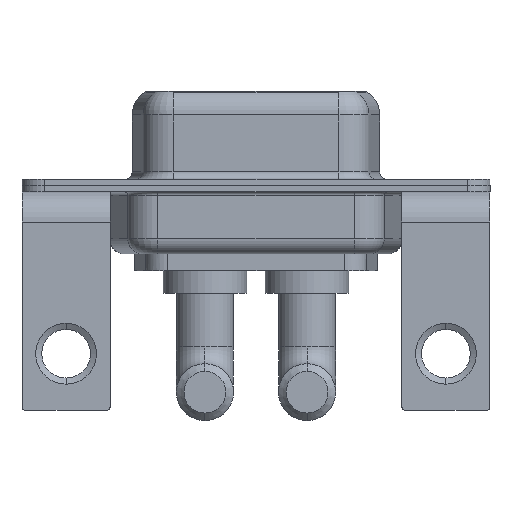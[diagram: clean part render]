
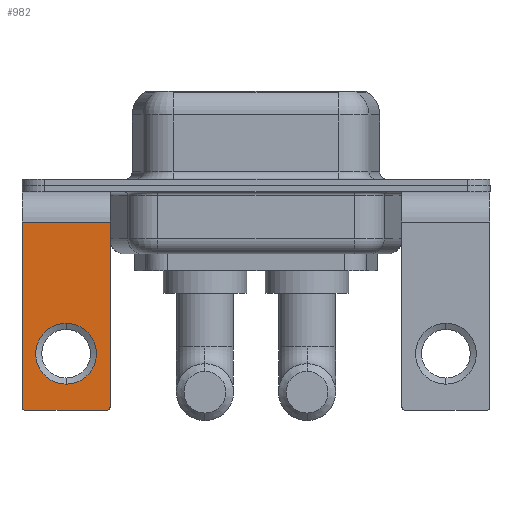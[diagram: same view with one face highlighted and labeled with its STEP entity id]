
A CAD part, front view. The second image highlights one B-rep face of the part: STEP entity #982.
In plain terms, the highlighted planar face has unit normal (0, -1, 0).
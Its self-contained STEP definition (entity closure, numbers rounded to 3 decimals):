
#19 = VERTEX_POINT ( 'NONE', #1839 ) ;
#509 = VECTOR ( 'NONE', #10848, 1000. ) ;
#629 = LINE ( 'NONE', #2600, #3010 ) ;
#982 = ADVANCED_FACE ( 'NONE', ( #2645, #2837 ), #10839, .F. ) ;
#1066 = ORIENTED_EDGE ( 'NONE', *, *, #7491, .F. ) ;
#1221 = ORIENTED_EDGE ( 'NONE', *, *, #5787, .T. ) ;
#1778 = EDGE_LOOP ( 'NONE', ( #9861, #5299, #6049, #1221, #1066, #8559 ) ) ;
#1783 = DIRECTION ( 'NONE',  ( 0., 1., 0. ) ) ;
#1839 = CARTESIAN_POINT ( 'NONE',  ( -2.9, -6.25, -2.4 ) ) ;
#1946 = CARTESIAN_POINT ( 'NONE',  ( 2.65, -6.25, -14.55 ) ) ;
#2063 = DIRECTION ( 'NONE',  ( 0., 0., 1. ) ) ;
#2127 = DIRECTION ( 'NONE',  ( -1., 0., 0. ) ) ;
#2351 = CARTESIAN_POINT ( 'NONE',  ( 0., -6.25, -11.07 ) ) ;
#2417 = CARTESIAN_POINT ( 'NONE',  ( -2.9, -6.25, -14.55 ) ) ;
#2541 = CARTESIAN_POINT ( 'NONE',  ( 2.9, -6.25, -14.55 ) ) ;
#2587 = EDGE_CURVE ( 'NONE', #19, #12319, #629, .T. ) ;
#2600 = CARTESIAN_POINT ( 'NONE',  ( -2.9, -6.25, -2.4 ) ) ;
#2645 = FACE_BOUND ( 'NONE', #3706, .T. ) ;
#2831 = CARTESIAN_POINT ( 'NONE',  ( 0., -6.25, -13.07 ) ) ;
#2837 = FACE_OUTER_BOUND ( 'NONE', #1778, .T. ) ;
#3010 = VECTOR ( 'NONE', #6517, 1000. ) ;
#3052 = DIRECTION ( 'NONE',  ( 0., -1., 0. ) ) ;
#3208 = CIRCLE ( 'NONE', #12373, 0.25 ) ;
#3221 = LINE ( 'NONE', #9207, #9696 ) ;
#3277 = AXIS2_PLACEMENT_3D ( 'NONE', #2351, #10372, #4375 ) ;
#3706 = EDGE_LOOP ( 'NONE', ( #7276, #4104 ) ) ;
#4031 = CARTESIAN_POINT ( 'NONE',  ( -2.65, -6.25, -14.55 ) ) ;
#4104 = ORIENTED_EDGE ( 'NONE', *, *, #11222, .T. ) ;
#4375 = DIRECTION ( 'NONE',  ( 0., 0., 1. ) ) ;
#5279 = CIRCLE ( 'NONE', #9665, 0.25 ) ;
#5299 = ORIENTED_EDGE ( 'NONE', *, *, #6335, .T. ) ;
#5304 = DIRECTION ( 'NONE',  ( 0., 0., -1. ) ) ;
#5578 = VERTEX_POINT ( 'NONE', #2541 ) ;
#5787 = EDGE_CURVE ( 'NONE', #9350, #5578, #5279, .T. ) ;
#5809 = CIRCLE ( 'NONE', #6012, 2. ) ;
#5944 = DIRECTION ( 'NONE',  ( 0., 0., 1. ) ) ;
#5954 = VECTOR ( 'NONE', #2127, 1000. ) ;
#6006 = CARTESIAN_POINT ( 'NONE',  ( -2.65, -6.25, -14.8 ) ) ;
#6012 = AXIS2_PLACEMENT_3D ( 'NONE', #11103, #6037, #7072 ) ;
#6037 = DIRECTION ( 'NONE',  ( 0., 1., 0. ) ) ;
#6049 = ORIENTED_EDGE ( 'NONE', *, *, #7111, .F. ) ;
#6335 = EDGE_CURVE ( 'NONE', #12319, #8332, #3208, .T. ) ;
#6382 = LINE ( 'NONE', #11058, #5954 ) ;
#6517 = DIRECTION ( 'NONE',  ( 0., 0., -1. ) ) ;
#6741 = EDGE_CURVE ( 'NONE', #12551, #19, #8906, .T. ) ;
#6819 = DIRECTION ( 'NONE',  ( 0., 0., 1. ) ) ;
#7072 = DIRECTION ( 'NONE',  ( 0., 0., 1. ) ) ;
#7111 = EDGE_CURVE ( 'NONE', #9350, #8332, #6382, .T. ) ;
#7276 = ORIENTED_EDGE ( 'NONE', *, *, #12384, .T. ) ;
#7491 = EDGE_CURVE ( 'NONE', #12551, #5578, #3221, .T. ) ;
#7891 = CARTESIAN_POINT ( 'NONE',  ( 2.9, -6.25, -2.4 ) ) ;
#8287 = CARTESIAN_POINT ( 'NONE',  ( 2.9, -6.25, -2.4 ) ) ;
#8332 = VERTEX_POINT ( 'NONE', #6006 ) ;
#8559 = ORIENTED_EDGE ( 'NONE', *, *, #6741, .T. ) ;
#8906 = LINE ( 'NONE', #8287, #509 ) ;
#9146 = VERTEX_POINT ( 'NONE', #2831 ) ;
#9207 = CARTESIAN_POINT ( 'NONE',  ( 2.9, -6.25, -2.4 ) ) ;
#9262 = CARTESIAN_POINT ( 'NONE',  ( 0., -6.25, -9.07 ) ) ;
#9350 = VERTEX_POINT ( 'NONE', #12330 ) ;
#9665 = AXIS2_PLACEMENT_3D ( 'NONE', #1946, #11738, #5944 ) ;
#9686 = CARTESIAN_POINT ( 'NONE',  ( 2.9, -6.25, -2.4 ) ) ;
#9696 = VECTOR ( 'NONE', #5304, 1000. ) ;
#9861 = ORIENTED_EDGE ( 'NONE', *, *, #2587, .T. ) ;
#10348 = CIRCLE ( 'NONE', #3277, 2. ) ;
#10372 = DIRECTION ( 'NONE',  ( 0., 1., 0. ) ) ;
#10839 = PLANE ( 'NONE',  #10877 ) ;
#10848 = DIRECTION ( 'NONE',  ( -1., 0., 0. ) ) ;
#10877 = AXIS2_PLACEMENT_3D ( 'NONE', #9686, #1783, #6819 ) ;
#11058 = CARTESIAN_POINT ( 'NONE',  ( 2.9, -6.25, -14.8 ) ) ;
#11103 = CARTESIAN_POINT ( 'NONE',  ( 0., -6.25, -11.07 ) ) ;
#11222 = EDGE_CURVE ( 'NONE', #12060, #9146, #5809, .T. ) ;
#11738 = DIRECTION ( 'NONE',  ( 0., -1., 0. ) ) ;
#12060 = VERTEX_POINT ( 'NONE', #9262 ) ;
#12319 = VERTEX_POINT ( 'NONE', #2417 ) ;
#12330 = CARTESIAN_POINT ( 'NONE',  ( 2.65, -6.25, -14.8 ) ) ;
#12373 = AXIS2_PLACEMENT_3D ( 'NONE', #4031, #3052, #2063 ) ;
#12384 = EDGE_CURVE ( 'NONE', #9146, #12060, #10348, .T. ) ;
#12551 = VERTEX_POINT ( 'NONE', #7891 ) ;
